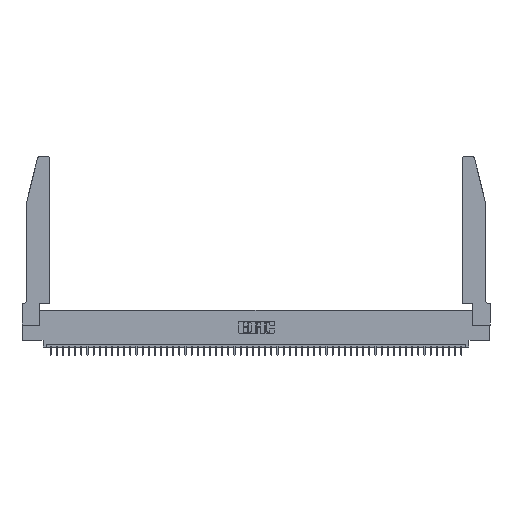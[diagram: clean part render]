
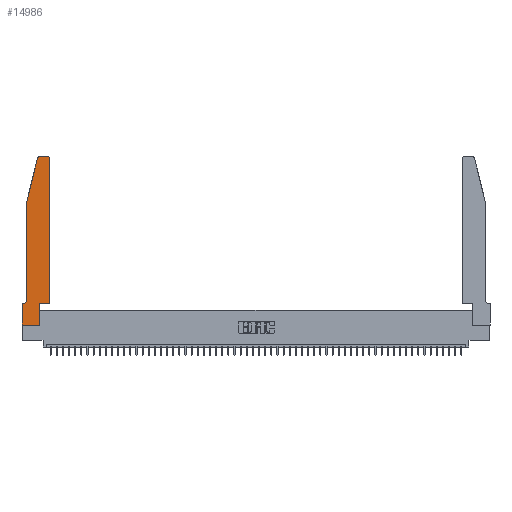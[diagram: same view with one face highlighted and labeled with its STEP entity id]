
A CAD part, top view. The second image highlights one B-rep face of the part: STEP entity #14986.
In plain terms, the highlighted planar face has unit normal (0, 0, 1).
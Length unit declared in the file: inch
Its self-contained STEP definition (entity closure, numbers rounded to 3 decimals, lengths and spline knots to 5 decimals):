
#438 = ORIENTED_EDGE ( 'NONE', *, *, #28549, .T. ) ;
#1342 = CIRCLE ( 'NONE', #53689, 0.03 ) ;
#1485 = DIRECTION ( 'NONE',  ( -1., 0., 0. ) ) ;
#1882 = VECTOR ( 'NONE', #47445, 39.37008 ) ;
#2001 = LINE ( 'NONE', #52559, #54397 ) ;
#2332 = VERTEX_POINT ( 'NONE', #40489 ) ;
#2337 = LINE ( 'NONE', #14558, #37810 ) ;
#2541 = LINE ( 'NONE', #19194, #12529 ) ;
#2710 = EDGE_CURVE ( 'NONE', #12624, #2332, #48475, .T. ) ;
#3092 = EDGE_CURVE ( 'NONE', #7335, #49586, #19450, .T. ) ;
#3341 = CARTESIAN_POINT ( 'NONE',  ( 0.284, 2.75, 0.37 ) ) ;
#3376 = ORIENTED_EDGE ( 'NONE', *, *, #26369, .T. ) ;
#4243 = DIRECTION ( 'NONE',  ( 0., 0., 1. ) ) ;
#4807 = DIRECTION ( 'NONE',  ( 1., 0., 0. ) ) ;
#4827 = CARTESIAN_POINT ( 'NONE',  ( 0., 0., 0.37 ) ) ;
#5401 = EDGE_CURVE ( 'NONE', #18597, #31040, #2337, .T. ) ;
#6174 = LINE ( 'NONE', #22826, #53515 ) ;
#6563 = DIRECTION ( 'NONE',  ( 1., 0., 0. ) ) ;
#7335 = VERTEX_POINT ( 'NONE', #14758 ) ;
#9522 = EDGE_CURVE ( 'NONE', #47981, #50080, #10496, .T. ) ;
#10138 = LINE ( 'NONE', #47888, #32081 ) ;
#10496 = CIRCLE ( 'NONE', #14049, 0.07 ) ;
#10667 = DIRECTION ( 'NONE',  ( -1., 0., 0. ) ) ;
#11086 = ORIENTED_EDGE ( 'NONE', *, *, #15912, .T. ) ;
#11202 = CARTESIAN_POINT ( 'NONE',  ( 0.4505, 2.72, 0.37 ) ) ;
#12300 = CARTESIAN_POINT ( 'NONE',  ( 0., 0.35, 0.37 ) ) ;
#12323 = ORIENTED_EDGE ( 'NONE', *, *, #5401, .T. ) ;
#12529 = VECTOR ( 'NONE', #49189, 39.37008 ) ;
#12609 = ORIENTED_EDGE ( 'NONE', *, *, #3092, .T. ) ;
#12624 = VERTEX_POINT ( 'NONE', #54090 ) ;
#12669 = DIRECTION ( 'NONE',  ( 0., 0., 1. ) ) ;
#12836 = VECTOR ( 'NONE', #1485, 39.37008 ) ;
#14049 = AXIS2_PLACEMENT_3D ( 'NONE', #23360, #15854, #19197 ) ;
#14053 = CARTESIAN_POINT ( 'NONE',  ( 0.4505, 0.35, 0.37 ) ) ;
#14271 = DIRECTION ( 'NONE',  ( 0., -1., 0. ) ) ;
#14558 = CARTESIAN_POINT ( 'NONE',  ( 0., 0., 0.37 ) ) ;
#14758 = CARTESIAN_POINT ( 'NONE',  ( 0.4205, 2.75, 0.37 ) ) ;
#14986 = ADVANCED_FACE ( 'NONE', ( #16464 ), #37841, .T. ) ;
#15253 = EDGE_CURVE ( 'NONE', #41746, #12624, #2541, .T. ) ;
#15854 = DIRECTION ( 'NONE',  ( 0., 0., -1. ) ) ;
#15900 = EDGE_CURVE ( 'NONE', #50080, #18597, #31213, .T. ) ;
#15912 = EDGE_CURVE ( 'NONE', #32677, #26859, #10138, .T. ) ;
#16464 = FACE_OUTER_BOUND ( 'NONE', #27004, .T. ) ;
#16907 = EDGE_CURVE ( 'NONE', #49586, #32677, #28749, .T. ) ;
#16967 = DIRECTION ( 'NONE',  ( 0., 0., 1. ) ) ;
#17668 = DIRECTION ( 'NONE',  ( 1., 0., 0. ) ) ;
#18373 = ORIENTED_EDGE ( 'NONE', *, *, #2710, .T. ) ;
#18597 = VERTEX_POINT ( 'NONE', #41326 ) ;
#18942 = DIRECTION ( 'NONE',  ( 0., 1., 0. ) ) ;
#19093 = ORIENTED_EDGE ( 'NONE', *, *, #44740, .T. ) ;
#19194 = CARTESIAN_POINT ( 'NONE',  ( 0.2865, 0.35, 0.37 ) ) ;
#19197 = DIRECTION ( 'NONE',  ( -1., 0., 0. ) ) ;
#19252 = CARTESIAN_POINT ( 'NONE',  ( 0.0755, 0.42, 0.37 ) ) ;
#19450 = LINE ( 'NONE', #23890, #12836 ) ;
#21964 = ORIENTED_EDGE ( 'NONE', *, *, #16907, .T. ) ;
#22826 = CARTESIAN_POINT ( 'NONE',  ( 0.0755, 2., 0.37 ) ) ;
#23360 = CARTESIAN_POINT ( 'NONE',  ( 0.0055, 0.42, 0.37 ) ) ;
#23890 = CARTESIAN_POINT ( 'NONE',  ( 0.2605, 2.75, 0.37 ) ) ;
#26048 = ORIENTED_EDGE ( 'NONE', *, *, #15900, .T. ) ;
#26369 = EDGE_CURVE ( 'NONE', #31040, #41746, #42447, .T. ) ;
#26859 = VERTEX_POINT ( 'NONE', #34054 ) ;
#26946 = AXIS2_PLACEMENT_3D ( 'NONE', #50728, #12669, #17668 ) ;
#27004 = EDGE_LOOP ( 'NONE', ( #12609, #21964, #11086, #438, #40202, #26048, #12323, #3376, #48173, #18373, #29342, #19093 ) ) ;
#27601 = AXIS2_PLACEMENT_3D ( 'NONE', #12300, #4243, #4807 ) ;
#28549 = EDGE_CURVE ( 'NONE', #26859, #47981, #6174, .T. ) ;
#28585 = EDGE_CURVE ( 'NONE', #2332, #39048, #2001, .T. ) ;
#28749 = CIRCLE ( 'NONE', #26946, 0.03 ) ;
#29342 = ORIENTED_EDGE ( 'NONE', *, *, #28585, .T. ) ;
#29484 = DIRECTION ( 'NONE',  ( 1., 0., 0. ) ) ;
#31040 = VERTEX_POINT ( 'NONE', #4827 ) ;
#31213 = LINE ( 'NONE', #39558, #47186 ) ;
#32081 = VECTOR ( 'NONE', #35387, 39.37008 ) ;
#32677 = VERTEX_POINT ( 'NONE', #41173 ) ;
#34054 = CARTESIAN_POINT ( 'NONE',  ( 0.0755, 2., 0.37 ) ) ;
#35387 = DIRECTION ( 'NONE',  ( -0.239, -0.971, 0. ) ) ;
#37810 = VECTOR ( 'NONE', #14271, 39.37008 ) ;
#37841 = PLANE ( 'NONE',  #27601 ) ;
#39048 = VERTEX_POINT ( 'NONE', #11202 ) ;
#39558 = CARTESIAN_POINT ( 'NONE',  ( 0.0755, 0.35, 0.37 ) ) ;
#39569 = VECTOR ( 'NONE', #6563, 39.37008 ) ;
#40202 = ORIENTED_EDGE ( 'NONE', *, *, #9522, .T. ) ;
#40489 = CARTESIAN_POINT ( 'NONE',  ( 0.4505, 0.35, 0.37 ) ) ;
#41173 = CARTESIAN_POINT ( 'NONE',  ( 0.25487, 2.72718, 0.37 ) ) ;
#41315 = CARTESIAN_POINT ( 'NONE',  ( 0.0055, 0.35, 0.37 ) ) ;
#41326 = CARTESIAN_POINT ( 'NONE',  ( 0., 0.35, 0.37 ) ) ;
#41746 = VERTEX_POINT ( 'NONE', #52284 ) ;
#42447 = LINE ( 'NONE', #51634, #1882 ) ;
#42806 = CARTESIAN_POINT ( 'NONE',  ( 0.4205, 2.72, 0.37 ) ) ;
#44472 = DIRECTION ( 'NONE',  ( 0., -1., 0. ) ) ;
#44740 = EDGE_CURVE ( 'NONE', #39048, #7335, #1342, .T. ) ;
#47186 = VECTOR ( 'NONE', #10667, 39.37008 ) ;
#47445 = DIRECTION ( 'NONE',  ( 1., 0., 0. ) ) ;
#47888 = CARTESIAN_POINT ( 'NONE',  ( 0.0755, 2., 0.37 ) ) ;
#47981 = VERTEX_POINT ( 'NONE', #19252 ) ;
#48173 = ORIENTED_EDGE ( 'NONE', *, *, #15253, .T. ) ;
#48475 = LINE ( 'NONE', #14053, #39569 ) ;
#49189 = DIRECTION ( 'NONE',  ( 0., 1., 0. ) ) ;
#49586 = VERTEX_POINT ( 'NONE', #3341 ) ;
#50080 = VERTEX_POINT ( 'NONE', #41315 ) ;
#50728 = CARTESIAN_POINT ( 'NONE',  ( 0.284, 2.72, 0.37 ) ) ;
#51634 = CARTESIAN_POINT ( 'NONE',  ( 0., 0., 0.37 ) ) ;
#52284 = CARTESIAN_POINT ( 'NONE',  ( 0.2865, 0., 0.37 ) ) ;
#52559 = CARTESIAN_POINT ( 'NONE',  ( 0.4505, 0.35, 0.37 ) ) ;
#53515 = VECTOR ( 'NONE', #44472, 39.37008 ) ;
#53689 = AXIS2_PLACEMENT_3D ( 'NONE', #42806, #16967, #29484 ) ;
#54090 = CARTESIAN_POINT ( 'NONE',  ( 0.2865, 0.35, 0.37 ) ) ;
#54397 = VECTOR ( 'NONE', #18942, 39.37008 ) ;
